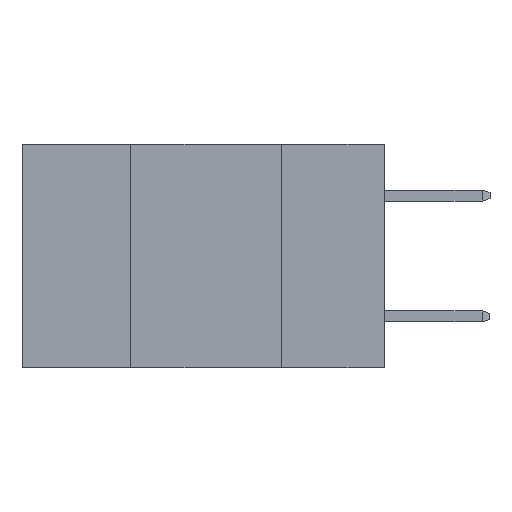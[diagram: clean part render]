
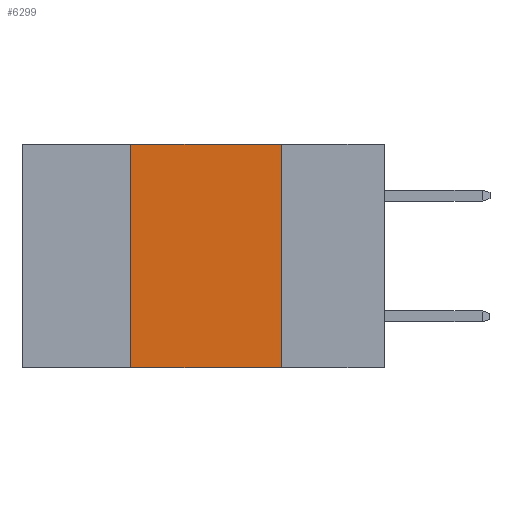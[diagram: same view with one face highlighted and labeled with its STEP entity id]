
A CAD part, left-side view. The second image highlights one B-rep face of the part: STEP entity #6299.
In plain terms, the highlighted planar face has unit normal (-1, 0, 0).
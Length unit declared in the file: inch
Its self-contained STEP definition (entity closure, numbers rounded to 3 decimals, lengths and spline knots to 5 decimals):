
#338 = ORIENTED_EDGE ( 'NONE', *, *, #16124, .F. ) ;
#369 = CARTESIAN_POINT ( 'NONE',  ( 0., 0.6, 0. ) ) ;
#635 = EDGE_CURVE ( 'NONE', #2310, #958, #15985, .T. ) ;
#958 = VERTEX_POINT ( 'NONE', #7629 ) ;
#1385 = DIRECTION ( 'NONE',  ( 0., 0., -1. ) ) ;
#1542 = CARTESIAN_POINT ( 'NONE',  ( 0., 0.17, 0. ) ) ;
#1716 = DIRECTION ( 'NONE',  ( 0., 0., -1. ) ) ;
#2310 = VERTEX_POINT ( 'NONE', #8517 ) ;
#4027 = VECTOR ( 'NONE', #9438, 39.37008 ) ;
#4421 = FACE_OUTER_BOUND ( 'NONE', #11986, .T. ) ;
#5171 = VECTOR ( 'NONE', #16178, 39.37008 ) ;
#5449 = AXIS2_PLACEMENT_3D ( 'NONE', #369, #9738, #1716 ) ;
#5635 = CARTESIAN_POINT ( 'NONE',  ( 0., 0.6, 0. ) ) ;
#6072 = ORIENTED_EDGE ( 'NONE', *, *, #13362, .F. ) ;
#6299 = ADVANCED_FACE ( 'NONE', ( #4421 ), #8426, .F. ) ;
#6836 = ORIENTED_EDGE ( 'NONE', *, *, #15334, .T. ) ;
#7561 = LINE ( 'NONE', #12007, #4027 ) ;
#7629 = CARTESIAN_POINT ( 'NONE',  ( 0., 0.17, -0.37 ) ) ;
#8426 = PLANE ( 'NONE',  #5449 ) ;
#8517 = CARTESIAN_POINT ( 'NONE',  ( 0., 0.17, 0. ) ) ;
#8943 = VECTOR ( 'NONE', #1385, 39.37008 ) ;
#9097 = LINE ( 'NONE', #5635, #5171 ) ;
#9354 = VERTEX_POINT ( 'NONE', #9492 ) ;
#9438 = DIRECTION ( 'NONE',  ( 0., 0., 1. ) ) ;
#9492 = CARTESIAN_POINT ( 'NONE',  ( 0., 0.42, -0.37 ) ) ;
#9738 = DIRECTION ( 'NONE',  ( 1., 0., 0. ) ) ;
#9852 = CARTESIAN_POINT ( 'NONE',  ( 0., 0.42, 0. ) ) ;
#10616 = ORIENTED_EDGE ( 'NONE', *, *, #635, .F. ) ;
#11610 = CARTESIAN_POINT ( 'NONE',  ( 0., 0.6, -0.37 ) ) ;
#11986 = EDGE_LOOP ( 'NONE', ( #10616, #6072, #338, #6836 ) ) ;
#12007 = CARTESIAN_POINT ( 'NONE',  ( 0., 0.42, 0. ) ) ;
#13362 = EDGE_CURVE ( 'NONE', #17003, #2310, #9097, .T. ) ;
#14721 = LINE ( 'NONE', #11610, #15109 ) ;
#15109 = VECTOR ( 'NONE', #15624, 39.37008 ) ;
#15334 = EDGE_CURVE ( 'NONE', #9354, #958, #14721, .T. ) ;
#15624 = DIRECTION ( 'NONE',  ( 0., -1., 0. ) ) ;
#15985 = LINE ( 'NONE', #1542, #8943 ) ;
#16124 = EDGE_CURVE ( 'NONE', #9354, #17003, #7561, .T. ) ;
#16178 = DIRECTION ( 'NONE',  ( 0., -1., 0. ) ) ;
#17003 = VERTEX_POINT ( 'NONE', #9852 ) ;
